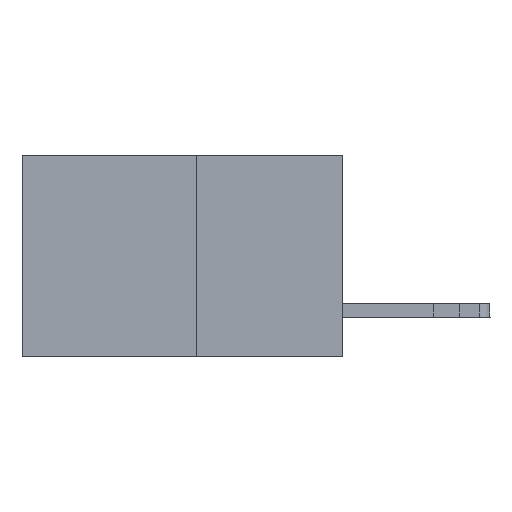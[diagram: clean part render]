
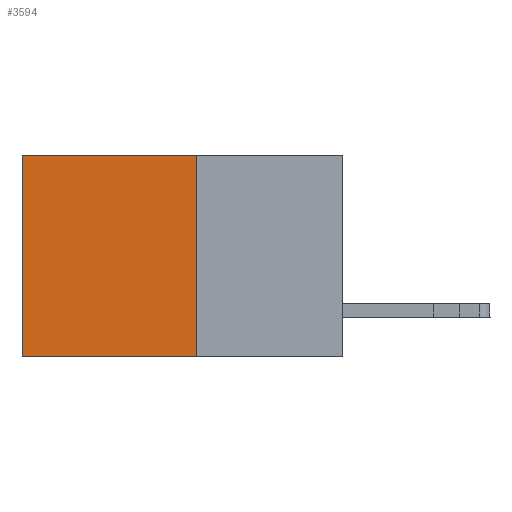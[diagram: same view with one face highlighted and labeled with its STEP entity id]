
A CAD part, left-side view. The second image highlights one B-rep face of the part: STEP entity #3594.
In plain terms, the highlighted planar face has unit normal (-1, 0, 0).
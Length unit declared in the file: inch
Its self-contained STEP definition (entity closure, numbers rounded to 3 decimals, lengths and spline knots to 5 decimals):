
#290 = EDGE_LOOP ( 'NONE', ( #14593, #1273, #8599, #6668 ) ) ;
#840 = VERTEX_POINT ( 'NONE', #14270 ) ;
#842 = CARTESIAN_POINT ( 'NONE',  ( 0.277, 0.59, -0.37 ) ) ;
#1008 = LINE ( 'NONE', #11615, #4498 ) ;
#1273 = ORIENTED_EDGE ( 'NONE', *, *, #1767, .F. ) ;
#1767 = EDGE_CURVE ( 'NONE', #6540, #3718, #4065, .T. ) ;
#1828 = DIRECTION ( 'NONE',  ( 0., 0., -1. ) ) ;
#3594 = ADVANCED_FACE ( 'NONE', ( #14305 ), #14281, .F. ) ;
#3637 = CARTESIAN_POINT ( 'NONE',  ( 0.277, 0.27, 0. ) ) ;
#3718 = VERTEX_POINT ( 'NONE', #842 ) ;
#4065 = LINE ( 'NONE', #14491, #14819 ) ;
#4296 = VERTEX_POINT ( 'NONE', #3637 ) ;
#4498 = VECTOR ( 'NONE', #12001, 39.37008 ) ;
#5087 = CARTESIAN_POINT ( 'NONE',  ( 0.277, 0.27, -0.37 ) ) ;
#6540 = VERTEX_POINT ( 'NONE', #5087 ) ;
#6668 = ORIENTED_EDGE ( 'NONE', *, *, #15061, .T. ) ;
#7021 = AXIS2_PLACEMENT_3D ( 'NONE', #14164, #16886, #1828 ) ;
#8265 = LINE ( 'NONE', #12868, #15160 ) ;
#8303 = EDGE_CURVE ( 'NONE', #4296, #6540, #1008, .T. ) ;
#8599 = ORIENTED_EDGE ( 'NONE', *, *, #8303, .F. ) ;
#8763 = DIRECTION ( 'NONE',  ( 0., 1., 0. ) ) ;
#9267 = LINE ( 'NONE', #9524, #14856 ) ;
#9524 = CARTESIAN_POINT ( 'NONE',  ( 0.277, 0.59, -0.37 ) ) ;
#11615 = CARTESIAN_POINT ( 'NONE',  ( 0.277, 0.27, -0.37 ) ) ;
#12001 = DIRECTION ( 'NONE',  ( 0., 0., -1. ) ) ;
#12293 = DIRECTION ( 'NONE',  ( 0., 0., -1. ) ) ;
#12868 = CARTESIAN_POINT ( 'NONE',  ( 0.277, 0.27, 0. ) ) ;
#13565 = EDGE_CURVE ( 'NONE', #840, #3718, #9267, .T. ) ;
#14164 = CARTESIAN_POINT ( 'NONE',  ( 0.277, 0.27, -0.37 ) ) ;
#14270 = CARTESIAN_POINT ( 'NONE',  ( 0.277, 0.59, 0. ) ) ;
#14281 = PLANE ( 'NONE',  #7021 ) ;
#14305 = FACE_OUTER_BOUND ( 'NONE', #290, .T. ) ;
#14491 = CARTESIAN_POINT ( 'NONE',  ( 0.277, 0.27, -0.37 ) ) ;
#14593 = ORIENTED_EDGE ( 'NONE', *, *, #13565, .T. ) ;
#14751 = DIRECTION ( 'NONE',  ( 0., 1., 0. ) ) ;
#14819 = VECTOR ( 'NONE', #14751, 39.37008 ) ;
#14856 = VECTOR ( 'NONE', #12293, 39.37008 ) ;
#15061 = EDGE_CURVE ( 'NONE', #4296, #840, #8265, .T. ) ;
#15160 = VECTOR ( 'NONE', #8763, 39.37008 ) ;
#16886 = DIRECTION ( 'NONE',  ( 1., 0., 0. ) ) ;
